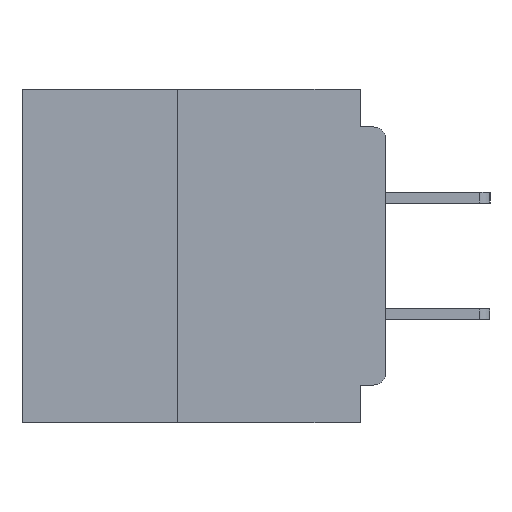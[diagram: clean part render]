
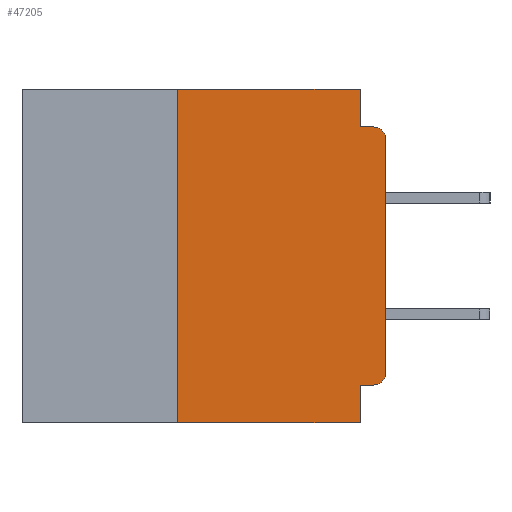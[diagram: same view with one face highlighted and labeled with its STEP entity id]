
A CAD part, left-side view. The second image highlights one B-rep face of the part: STEP entity #47205.
In plain terms, the highlighted planar face has unit normal (-1, 0, 0).
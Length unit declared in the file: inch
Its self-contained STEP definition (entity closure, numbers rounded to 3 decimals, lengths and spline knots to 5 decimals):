
#87 = CARTESIAN_POINT ( 'NONE',  ( 0., 0., -0.045 ) ) ;
#928 = ORIENTED_EDGE ( 'NONE', *, *, #19205, .T. ) ;
#1930 = LINE ( 'NONE', #31412, #9812 ) ;
#2133 = VECTOR ( 'NONE', #13790, 39.37008 ) ;
#3239 = ORIENTED_EDGE ( 'NONE', *, *, #25796, .T. ) ;
#4038 = EDGE_CURVE ( 'NONE', #48015, #28530, #8526, .T. ) ;
#4305 = CARTESIAN_POINT ( 'NONE',  ( 0., 0.031, 0. ) ) ;
#6097 = CIRCLE ( 'NONE', #45192, 0.015 ) ;
#7657 = DIRECTION ( 'NONE',  ( -1., 0., 0. ) ) ;
#8206 = DIRECTION ( 'NONE',  ( 0., 0., -1. ) ) ;
#8315 = LINE ( 'NONE', #14630, #47984 ) ;
#8526 = LINE ( 'NONE', #87, #17589 ) ;
#9302 = CARTESIAN_POINT ( 'NONE',  ( 0., 0.437, -0.4 ) ) ;
#9733 = CARTESIAN_POINT ( 'NONE',  ( 0., 0.015, -0.355 ) ) ;
#9812 = VECTOR ( 'NONE', #35290, 39.37008 ) ;
#10204 = EDGE_CURVE ( 'NONE', #12102, #49444, #49550, .T. ) ;
#11021 = AXIS2_PLACEMENT_3D ( 'NONE', #18013, #48714, #25829 ) ;
#11389 = VERTEX_POINT ( 'NONE', #13146 ) ;
#11466 = EDGE_CURVE ( 'NONE', #29659, #19353, #41660, .T. ) ;
#11982 = ORIENTED_EDGE ( 'NONE', *, *, #21842, .F. ) ;
#12102 = VERTEX_POINT ( 'NONE', #9733 ) ;
#12151 = VECTOR ( 'NONE', #40430, 39.37008 ) ;
#12732 = LINE ( 'NONE', #9302, #42231 ) ;
#12965 = DIRECTION ( 'NONE',  ( 0., 0., 1. ) ) ;
#13146 = CARTESIAN_POINT ( 'NONE',  ( 0., 0.25, 0. ) ) ;
#13199 = ORIENTED_EDGE ( 'NONE', *, *, #24439, .F. ) ;
#13790 = DIRECTION ( 'NONE',  ( 0., 0., 1. ) ) ;
#14630 = CARTESIAN_POINT ( 'NONE',  ( 0., 0.437, 0. ) ) ;
#15219 = CARTESIAN_POINT ( 'NONE',  ( 0., 0.031, -0.045 ) ) ;
#16354 = DIRECTION ( 'NONE',  ( -1., 0., 0. ) ) ;
#16504 = LINE ( 'NONE', #4305, #45944 ) ;
#17398 = ORIENTED_EDGE ( 'NONE', *, *, #10204, .T. ) ;
#17589 = VECTOR ( 'NONE', #46179, 39.37008 ) ;
#18013 = CARTESIAN_POINT ( 'NONE',  ( 0., 0.437, 0. ) ) ;
#18075 = CARTESIAN_POINT ( 'NONE',  ( 0., 0.031, -0.4 ) ) ;
#18815 = FACE_OUTER_BOUND ( 'NONE', #29047, .T. ) ;
#19205 = EDGE_CURVE ( 'NONE', #49650, #19353, #12732, .T. ) ;
#19353 = VERTEX_POINT ( 'NONE', #18075 ) ;
#20743 = CARTESIAN_POINT ( 'NONE',  ( 0., 0., 0. ) ) ;
#21722 = EDGE_CURVE ( 'NONE', #49444, #23603, #37818, .T. ) ;
#21803 = CARTESIAN_POINT ( 'NONE',  ( 0., 0., -0.06 ) ) ;
#21842 = EDGE_CURVE ( 'NONE', #49650, #11389, #43117, .T. ) ;
#23603 = VERTEX_POINT ( 'NONE', #21803 ) ;
#24439 = EDGE_CURVE ( 'NONE', #46976, #48015, #16504, .T. ) ;
#24864 = DIRECTION ( 'NONE',  ( 0., -1., 0. ) ) ;
#25347 = ORIENTED_EDGE ( 'NONE', *, *, #34273, .F. ) ;
#25487 = PLANE ( 'NONE',  #11021 ) ;
#25796 = EDGE_CURVE ( 'NONE', #23603, #28530, #6097, .T. ) ;
#25829 = DIRECTION ( 'NONE',  ( 0., 0., -1. ) ) ;
#27634 = VECTOR ( 'NONE', #12965, 39.37008 ) ;
#28405 = CARTESIAN_POINT ( 'NONE',  ( 0., 0.031, 0. ) ) ;
#28530 = VERTEX_POINT ( 'NONE', #39390 ) ;
#28929 = ORIENTED_EDGE ( 'NONE', *, *, #4038, .F. ) ;
#29047 = EDGE_LOOP ( 'NONE', ( #39526, #3239, #28929, #13199, #25347, #11982, #928, #47960, #39167, #17398 ) ) ;
#29185 = CARTESIAN_POINT ( 'NONE',  ( 0., 0.25, -0.4 ) ) ;
#29659 = VERTEX_POINT ( 'NONE', #35162 ) ;
#30843 = CARTESIAN_POINT ( 'NONE',  ( 0., 0.015, -0.34 ) ) ;
#30958 = EDGE_CURVE ( 'NONE', #12102, #29659, #1930, .T. ) ;
#31412 = CARTESIAN_POINT ( 'NONE',  ( 0., 0., -0.355 ) ) ;
#32590 = AXIS2_PLACEMENT_3D ( 'NONE', #30843, #7657, #34714 ) ;
#34273 = EDGE_CURVE ( 'NONE', #11389, #46976, #8315, .T. ) ;
#34714 = DIRECTION ( 'NONE',  ( 0., 0., -1. ) ) ;
#35162 = CARTESIAN_POINT ( 'NONE',  ( 0., 0.031, -0.355 ) ) ;
#35290 = DIRECTION ( 'NONE',  ( 0., 1., 0. ) ) ;
#35913 = CARTESIAN_POINT ( 'NONE',  ( 0., 0., -0.34 ) ) ;
#36942 = CARTESIAN_POINT ( 'NONE',  ( 0., 0.25, -0.4 ) ) ;
#37754 = DIRECTION ( 'NONE',  ( 0., -1., 0. ) ) ;
#37818 = LINE ( 'NONE', #20743, #27634 ) ;
#39167 = ORIENTED_EDGE ( 'NONE', *, *, #30958, .F. ) ;
#39390 = CARTESIAN_POINT ( 'NONE',  ( 0., 0.015, -0.045 ) ) ;
#39453 = CARTESIAN_POINT ( 'NONE',  ( 0., 0.015, -0.06 ) ) ;
#39526 = ORIENTED_EDGE ( 'NONE', *, *, #21722, .T. ) ;
#40430 = DIRECTION ( 'NONE',  ( 0., 0., -1. ) ) ;
#40597 = CARTESIAN_POINT ( 'NONE',  ( 0., 0.031, -0.4 ) ) ;
#41660 = LINE ( 'NONE', #40597, #12151 ) ;
#42231 = VECTOR ( 'NONE', #24864, 39.37008 ) ;
#43117 = LINE ( 'NONE', #36942, #2133 ) ;
#43239 = DIRECTION ( 'NONE',  ( 0., 0., -1. ) ) ;
#45192 = AXIS2_PLACEMENT_3D ( 'NONE', #39453, #16354, #43239 ) ;
#45944 = VECTOR ( 'NONE', #8206, 39.37008 ) ;
#46179 = DIRECTION ( 'NONE',  ( 0., -1., 0. ) ) ;
#46976 = VERTEX_POINT ( 'NONE', #28405 ) ;
#47205 = ADVANCED_FACE ( 'NONE', ( #18815 ), #25487, .F. ) ;
#47960 = ORIENTED_EDGE ( 'NONE', *, *, #11466, .F. ) ;
#47984 = VECTOR ( 'NONE', #37754, 39.37008 ) ;
#48015 = VERTEX_POINT ( 'NONE', #15219 ) ;
#48714 = DIRECTION ( 'NONE',  ( 1., 0., 0. ) ) ;
#49444 = VERTEX_POINT ( 'NONE', #35913 ) ;
#49550 = CIRCLE ( 'NONE', #32590, 0.015 ) ;
#49650 = VERTEX_POINT ( 'NONE', #29185 ) ;
